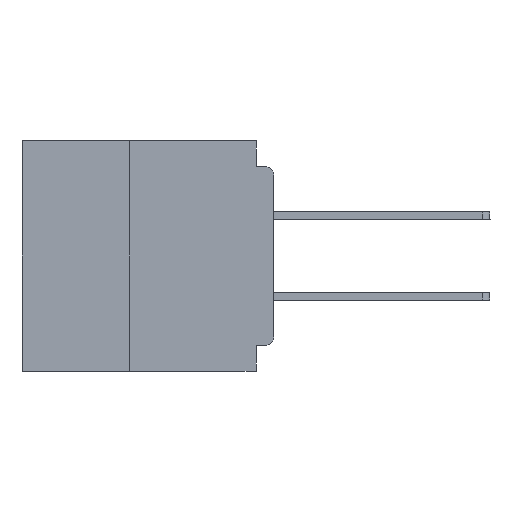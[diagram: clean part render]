
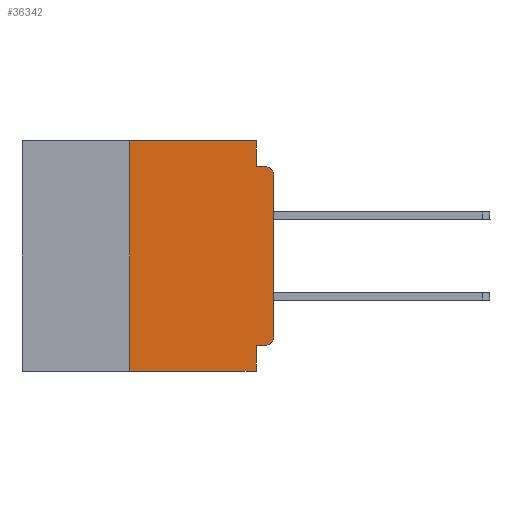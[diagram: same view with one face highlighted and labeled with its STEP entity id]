
A CAD part, left-side view. The second image highlights one B-rep face of the part: STEP entity #36342.
In plain terms, the highlighted planar face has unit normal (-1, 0, 0).
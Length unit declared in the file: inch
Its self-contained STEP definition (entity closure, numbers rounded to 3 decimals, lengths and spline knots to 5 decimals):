
#41 = CARTESIAN_POINT ( 'NONE',  ( 0., 0., -0.045 ) ) ;
#1238 = DIRECTION ( 'NONE',  ( 0., 0., -1. ) ) ;
#1763 = DIRECTION ( 'NONE',  ( 0., 0., -1. ) ) ;
#1999 = VERTEX_POINT ( 'NONE', #34390 ) ;
#2192 = VERTEX_POINT ( 'NONE', #18565 ) ;
#4573 = ORIENTED_EDGE ( 'NONE', *, *, #38870, .T. ) ;
#4853 = CARTESIAN_POINT ( 'NONE',  ( 0., 0., 0. ) ) ;
#5239 = DIRECTION ( 'NONE',  ( 0., -1., 0. ) ) ;
#5326 = FACE_OUTER_BOUND ( 'NONE', #12244, .T. ) ;
#5784 = ORIENTED_EDGE ( 'NONE', *, *, #34566, .F. ) ;
#6386 = LINE ( 'NONE', #39437, #32601 ) ;
#7430 = ORIENTED_EDGE ( 'NONE', *, *, #27760, .T. ) ;
#8026 = EDGE_CURVE ( 'NONE', #2192, #9458, #6386, .T. ) ;
#8180 = VERTEX_POINT ( 'NONE', #9249 ) ;
#9249 = CARTESIAN_POINT ( 'NONE',  ( 0., 0.031, -0.4 ) ) ;
#9458 = VERTEX_POINT ( 'NONE', #15814 ) ;
#11220 = VERTEX_POINT ( 'NONE', #57380 ) ;
#11573 = VERTEX_POINT ( 'NONE', #39691 ) ;
#11872 = AXIS2_PLACEMENT_3D ( 'NONE', #27294, #32539, #1238 ) ;
#12117 = EDGE_CURVE ( 'NONE', #48343, #58146, #23817, .T. ) ;
#12244 = EDGE_LOOP ( 'NONE', ( #43866, #65162, #18273, #64197, #41694, #22835, #7430, #5784, #36723, #4573 ) ) ;
#13982 = DIRECTION ( 'NONE',  ( 0., -1., 0. ) ) ;
#14229 = VECTOR ( 'NONE', #28206, 39.37008 ) ;
#15107 = EDGE_CURVE ( 'NONE', #9458, #58146, #53770, .T. ) ;
#15746 = DIRECTION ( 'NONE',  ( -1., 0., 0. ) ) ;
#15814 = CARTESIAN_POINT ( 'NONE',  ( 0., 0.031, -0.045 ) ) ;
#17716 = AXIS2_PLACEMENT_3D ( 'NONE', #46919, #15746, #52140 ) ;
#18273 = ORIENTED_EDGE ( 'NONE', *, *, #15107, .F. ) ;
#18565 = CARTESIAN_POINT ( 'NONE',  ( 0., 0.031, 0. ) ) ;
#18925 = DIRECTION ( 'NONE',  ( 0., -1., 0. ) ) ;
#19551 = CARTESIAN_POINT ( 'NONE',  ( 0., 0., -0.06 ) ) ;
#21190 = LINE ( 'NONE', #33081, #35068 ) ;
#21759 = EDGE_CURVE ( 'NONE', #11573, #2192, #55153, .T. ) ;
#22835 = ORIENTED_EDGE ( 'NONE', *, *, #61465, .F. ) ;
#23272 = EDGE_CURVE ( 'NONE', #32693, #11220, #29762, .T. ) ;
#23432 = CARTESIAN_POINT ( 'NONE',  ( 0., 0.015, -0.06 ) ) ;
#23817 = CIRCLE ( 'NONE', #55903, 0.015 ) ;
#24271 = CARTESIAN_POINT ( 'NONE',  ( 0., 0.437, -0.4 ) ) ;
#24436 = CARTESIAN_POINT ( 'NONE',  ( 0., 0.015, -0.045 ) ) ;
#24532 = VECTOR ( 'NONE', #5239, 39.37008 ) ;
#27294 = CARTESIAN_POINT ( 'NONE',  ( 0., 0.437, 0. ) ) ;
#27760 = EDGE_CURVE ( 'NONE', #1999, #8180, #32215, .T. ) ;
#28206 = DIRECTION ( 'NONE',  ( 0., 1., 0. ) ) ;
#28671 = DIRECTION ( 'NONE',  ( 0., 0., -1. ) ) ;
#29762 = LINE ( 'NONE', #48834, #14229 ) ;
#32215 = LINE ( 'NONE', #24271, #58158 ) ;
#32539 = DIRECTION ( 'NONE',  ( 1., 0., 0. ) ) ;
#32601 = VECTOR ( 'NONE', #65212, 39.37008 ) ;
#32693 = VERTEX_POINT ( 'NONE', #53218 ) ;
#33081 = CARTESIAN_POINT ( 'NONE',  ( 0., 0.031, -0.4 ) ) ;
#34390 = CARTESIAN_POINT ( 'NONE',  ( 0., 0.25, -0.4 ) ) ;
#34566 = EDGE_CURVE ( 'NONE', #11220, #8180, #21190, .T. ) ;
#35068 = VECTOR ( 'NONE', #1763, 39.37008 ) ;
#35993 = LINE ( 'NONE', #63771, #61905 ) ;
#36342 = ADVANCED_FACE ( 'NONE', ( #5326 ), #58372, .F. ) ;
#36723 = ORIENTED_EDGE ( 'NONE', *, *, #23272, .F. ) ;
#37976 = CARTESIAN_POINT ( 'NONE',  ( 0., 0., -0.34 ) ) ;
#38870 = EDGE_CURVE ( 'NONE', #32693, #40262, #61990, .T. ) ;
#39437 = CARTESIAN_POINT ( 'NONE',  ( 0., 0.031, 0. ) ) ;
#39691 = CARTESIAN_POINT ( 'NONE',  ( 0., 0.25, 0. ) ) ;
#39698 = CARTESIAN_POINT ( 'NONE',  ( 0., 0.437, 0. ) ) ;
#40262 = VERTEX_POINT ( 'NONE', #37976 ) ;
#41414 = DIRECTION ( 'NONE',  ( 0., 0., 1. ) ) ;
#41694 = ORIENTED_EDGE ( 'NONE', *, *, #21759, .F. ) ;
#43143 = DIRECTION ( 'NONE',  ( 0., 0., 1. ) ) ;
#43866 = ORIENTED_EDGE ( 'NONE', *, *, #53862, .T. ) ;
#45368 = LINE ( 'NONE', #4853, #59139 ) ;
#46919 = CARTESIAN_POINT ( 'NONE',  ( 0., 0.015, -0.34 ) ) ;
#48343 = VERTEX_POINT ( 'NONE', #19551 ) ;
#48834 = CARTESIAN_POINT ( 'NONE',  ( 0., 0., -0.355 ) ) ;
#52140 = DIRECTION ( 'NONE',  ( 0., 0., -1. ) ) ;
#53218 = CARTESIAN_POINT ( 'NONE',  ( 0., 0.015, -0.355 ) ) ;
#53505 = VECTOR ( 'NONE', #18925, 39.37008 ) ;
#53770 = LINE ( 'NONE', #41, #24532 ) ;
#53862 = EDGE_CURVE ( 'NONE', #40262, #48343, #45368, .T. ) ;
#55153 = LINE ( 'NONE', #39698, #53505 ) ;
#55903 = AXIS2_PLACEMENT_3D ( 'NONE', #23432, #59746, #28671 ) ;
#57380 = CARTESIAN_POINT ( 'NONE',  ( 0., 0.031, -0.355 ) ) ;
#58146 = VERTEX_POINT ( 'NONE', #24436 ) ;
#58158 = VECTOR ( 'NONE', #13982, 39.37008 ) ;
#58372 = PLANE ( 'NONE',  #11872 ) ;
#59139 = VECTOR ( 'NONE', #41414, 39.37008 ) ;
#59746 = DIRECTION ( 'NONE',  ( -1., 0., 0. ) ) ;
#61465 = EDGE_CURVE ( 'NONE', #1999, #11573, #35993, .T. ) ;
#61905 = VECTOR ( 'NONE', #43143, 39.37008 ) ;
#61990 = CIRCLE ( 'NONE', #17716, 0.015 ) ;
#63771 = CARTESIAN_POINT ( 'NONE',  ( 0., 0.25, -0.4 ) ) ;
#64197 = ORIENTED_EDGE ( 'NONE', *, *, #8026, .F. ) ;
#65162 = ORIENTED_EDGE ( 'NONE', *, *, #12117, .T. ) ;
#65212 = DIRECTION ( 'NONE',  ( 0., 0., -1. ) ) ;
